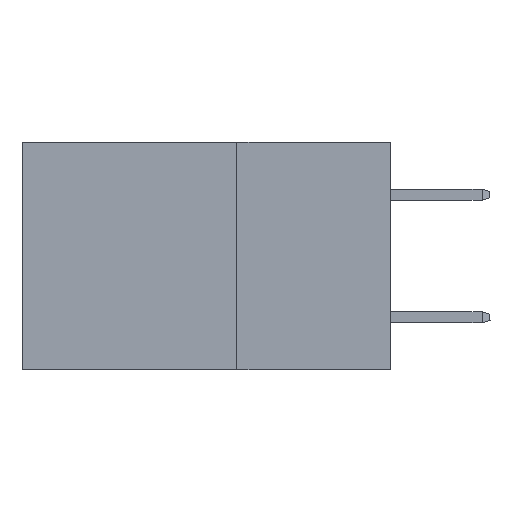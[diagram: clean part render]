
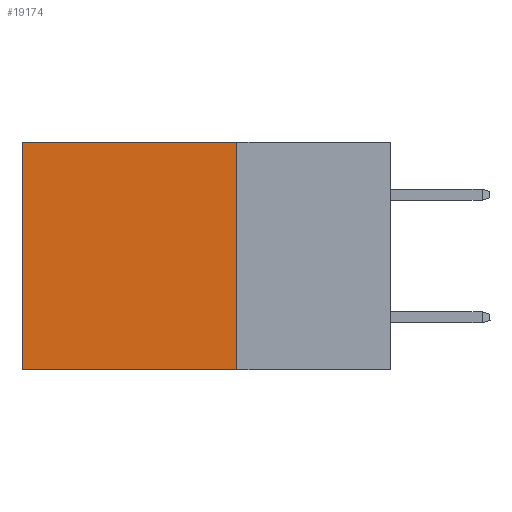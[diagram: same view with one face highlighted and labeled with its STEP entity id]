
A CAD part, left-side view. The second image highlights one B-rep face of the part: STEP entity #19174.
In plain terms, the highlighted planar face has unit normal (-1, 0, 0).
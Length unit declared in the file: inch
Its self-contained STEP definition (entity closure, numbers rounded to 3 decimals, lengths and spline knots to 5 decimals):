
#1037 = VERTEX_POINT ( 'NONE', #6508 ) ;
#2542 = VERTEX_POINT ( 'NONE', #40067 ) ;
#4016 = CARTESIAN_POINT ( 'NONE',  ( 0.2875, 0.25, 0. ) ) ;
#4110 = EDGE_CURVE ( 'NONE', #1037, #2542, #8816, .T. ) ;
#4538 = EDGE_CURVE ( 'NONE', #1037, #21583, #22509, .T. ) ;
#6360 = VECTOR ( 'NONE', #9988, 39.37008 ) ;
#6508 = CARTESIAN_POINT ( 'NONE',  ( 0.2875, 0.25, 0. ) ) ;
#8816 = LINE ( 'NONE', #14784, #17147 ) ;
#9931 = CARTESIAN_POINT ( 'NONE',  ( 0.2875, 0.25, -0.37 ) ) ;
#9988 = DIRECTION ( 'NONE',  ( 0., 1., 0. ) ) ;
#9990 = ORIENTED_EDGE ( 'NONE', *, *, #22269, .T. ) ;
#10579 = AXIS2_PLACEMENT_3D ( 'NONE', #37072, #18093, #18232 ) ;
#11186 = LINE ( 'NONE', #19459, #15132 ) ;
#11310 = CARTESIAN_POINT ( 'NONE',  ( 0.2875, 0.6, -0.37 ) ) ;
#11350 = DIRECTION ( 'NONE',  ( 0., 1., 0. ) ) ;
#14642 = VERTEX_POINT ( 'NONE', #11310 ) ;
#14784 = CARTESIAN_POINT ( 'NONE',  ( 0.2875, 0.25, 0. ) ) ;
#15132 = VECTOR ( 'NONE', #22775, 39.37008 ) ;
#15360 = PLANE ( 'NONE',  #10579 ) ;
#17147 = VECTOR ( 'NONE', #11350, 39.37008 ) ;
#18093 = DIRECTION ( 'NONE',  ( 1., 0., 0. ) ) ;
#18232 = DIRECTION ( 'NONE',  ( 0., 0., -1. ) ) ;
#18569 = ORIENTED_EDGE ( 'NONE', *, *, #39594, .F. ) ;
#18743 = ORIENTED_EDGE ( 'NONE', *, *, #4110, .T. ) ;
#19174 = ADVANCED_FACE ( 'NONE', ( #22213 ), #15360, .F. ) ;
#19459 = CARTESIAN_POINT ( 'NONE',  ( 0.2875, 0.6, 0. ) ) ;
#21583 = VERTEX_POINT ( 'NONE', #9931 ) ;
#22213 = FACE_OUTER_BOUND ( 'NONE', #37048, .T. ) ;
#22269 = EDGE_CURVE ( 'NONE', #2542, #14642, #11186, .T. ) ;
#22509 = LINE ( 'NONE', #4016, #26460 ) ;
#22741 = CARTESIAN_POINT ( 'NONE',  ( 0.2875, 0.25, -0.37 ) ) ;
#22775 = DIRECTION ( 'NONE',  ( 0., 0., -1. ) ) ;
#25993 = DIRECTION ( 'NONE',  ( 0., 0., -1. ) ) ;
#26460 = VECTOR ( 'NONE', #25993, 39.37008 ) ;
#32855 = ORIENTED_EDGE ( 'NONE', *, *, #4538, .F. ) ;
#37048 = EDGE_LOOP ( 'NONE', ( #9990, #18569, #32855, #18743 ) ) ;
#37072 = CARTESIAN_POINT ( 'NONE',  ( 0.2875, 0.25, 0. ) ) ;
#38958 = LINE ( 'NONE', #22741, #6360 ) ;
#39594 = EDGE_CURVE ( 'NONE', #21583, #14642, #38958, .T. ) ;
#40067 = CARTESIAN_POINT ( 'NONE',  ( 0.2875, 0.6, 0. ) ) ;
